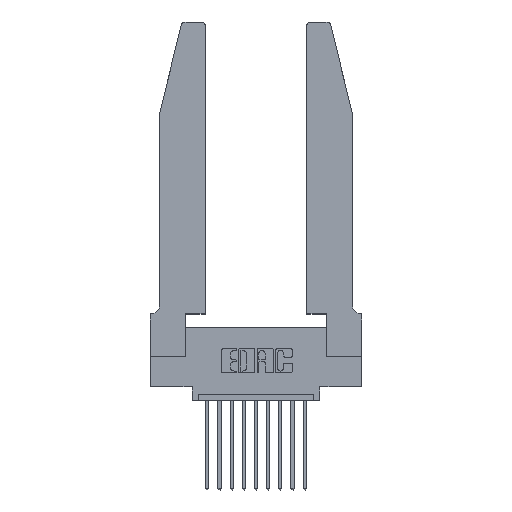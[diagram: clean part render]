
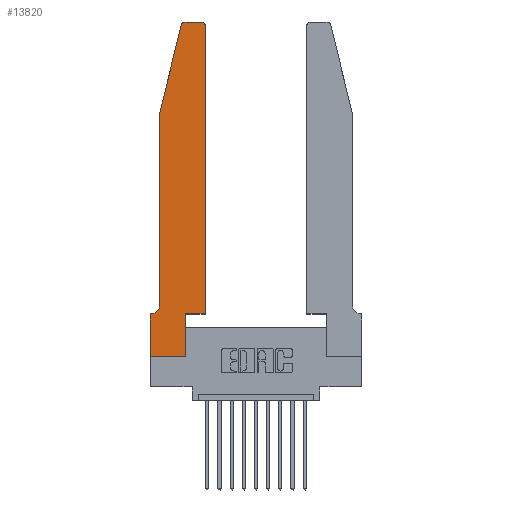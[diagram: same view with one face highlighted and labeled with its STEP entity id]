
A CAD part, top view. The second image highlights one B-rep face of the part: STEP entity #13820.
In plain terms, the highlighted planar face has unit normal (0, 0, 1).
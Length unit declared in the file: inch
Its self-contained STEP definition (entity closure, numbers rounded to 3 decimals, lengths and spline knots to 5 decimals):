
#143 = EDGE_CURVE ( 'NONE', #6618, #10646, #12908, .T. ) ;
#190 = ORIENTED_EDGE ( 'NONE', *, *, #7214, .T. ) ;
#289 = ORIENTED_EDGE ( 'NONE', *, *, #8067, .T. ) ;
#388 = CARTESIAN_POINT ( 'NONE',  ( 0.2865, 0.35, 0.37 ) ) ;
#455 = LINE ( 'NONE', #8012, #11568 ) ;
#609 = CARTESIAN_POINT ( 'NONE',  ( 0.0755, 2., 0.37 ) ) ;
#810 = LINE ( 'NONE', #609, #11160 ) ;
#1087 = VERTEX_POINT ( 'NONE', #6356 ) ;
#1095 = DIRECTION ( 'NONE',  ( -1., 0., 0. ) ) ;
#1259 = ORIENTED_EDGE ( 'NONE', *, *, #8394, .T. ) ;
#1332 = ORIENTED_EDGE ( 'NONE', *, *, #14107, .T. ) ;
#1530 = LINE ( 'NONE', #13356, #5033 ) ;
#1899 = EDGE_CURVE ( 'NONE', #15328, #15574, #11701, .T. ) ;
#1963 = VECTOR ( 'NONE', #5445, 39.37008 ) ;
#1976 = VECTOR ( 'NONE', #10586, 39.37008 ) ;
#2927 = CARTESIAN_POINT ( 'NONE',  ( 0.0055, 0.35, 0.37 ) ) ;
#2948 = ORIENTED_EDGE ( 'NONE', *, *, #13200, .T. ) ;
#3394 = EDGE_CURVE ( 'NONE', #10646, #1087, #8757, .T. ) ;
#3444 = ORIENTED_EDGE ( 'NONE', *, *, #10690, .T. ) ;
#3724 = CARTESIAN_POINT ( 'NONE',  ( 0.4205, 2.72, 0.37 ) ) ;
#3927 = VECTOR ( 'NONE', #7166, 39.37008 ) ;
#3982 = ORIENTED_EDGE ( 'NONE', *, *, #9500, .T. ) ;
#4256 = CARTESIAN_POINT ( 'NONE',  ( 0., 0., 0.37 ) ) ;
#4300 = CARTESIAN_POINT ( 'NONE',  ( 0.2605, 2.75, 0.37 ) ) ;
#4341 = ORIENTED_EDGE ( 'NONE', *, *, #1899, .T. ) ;
#4399 = VERTEX_POINT ( 'NONE', #6681 ) ;
#4404 = DIRECTION ( 'NONE',  ( -1., 0., 0. ) ) ;
#5033 = VECTOR ( 'NONE', #12233, 39.37008 ) ;
#5445 = DIRECTION ( 'NONE',  ( 0., 1., 0. ) ) ;
#5549 = VERTEX_POINT ( 'NONE', #4256 ) ;
#5720 = AXIS2_PLACEMENT_3D ( 'NONE', #7380, #11076, #8801 ) ;
#5830 = DIRECTION ( 'NONE',  ( 0., 0., 1. ) ) ;
#6044 = ORIENTED_EDGE ( 'NONE', *, *, #8778, .T. ) ;
#6047 = DIRECTION ( 'NONE',  ( 1., 0., 0. ) ) ;
#6051 = CARTESIAN_POINT ( 'NONE',  ( 0., 0.35, 0.37 ) ) ;
#6344 = CARTESIAN_POINT ( 'NONE',  ( 0.4505, 0.35, 0.37 ) ) ;
#6356 = CARTESIAN_POINT ( 'NONE',  ( 0.25487, 2.72718, 0.37 ) ) ;
#6618 = VERTEX_POINT ( 'NONE', #15232 ) ;
#6681 = CARTESIAN_POINT ( 'NONE',  ( 0.0755, 2., 0.37 ) ) ;
#6693 = DIRECTION ( 'NONE',  ( 1., 0., 0. ) ) ;
#6873 = VERTEX_POINT ( 'NONE', #14877 ) ;
#7014 = CARTESIAN_POINT ( 'NONE',  ( 0.0755, 0.42, 0.37 ) ) ;
#7020 = VERTEX_POINT ( 'NONE', #2927 ) ;
#7166 = DIRECTION ( 'NONE',  ( 1., 0., 0. ) ) ;
#7214 = EDGE_CURVE ( 'NONE', #4399, #14299, #810, .T. ) ;
#7265 = LINE ( 'NONE', #388, #7478 ) ;
#7380 = CARTESIAN_POINT ( 'NONE',  ( 0., 0.35, 0.37 ) ) ;
#7478 = VECTOR ( 'NONE', #10093, 39.37008 ) ;
#7617 = CIRCLE ( 'NONE', #12773, 0.03 ) ;
#7689 = EDGE_CURVE ( 'NONE', #7020, #16111, #13285, .T. ) ;
#7711 = VERTEX_POINT ( 'NONE', #15717 ) ;
#8012 = CARTESIAN_POINT ( 'NONE',  ( 0., 0., 0.37 ) ) ;
#8067 = EDGE_CURVE ( 'NONE', #7711, #15328, #9184, .T. ) ;
#8142 = CIRCLE ( 'NONE', #8944, 0.07 ) ;
#8385 = EDGE_LOOP ( 'NONE', ( #15115, #14340, #6044, #190, #3444, #8931, #3982, #1332, #2948, #289, #4341, #1259 ) ) ;
#8394 = EDGE_CURVE ( 'NONE', #15574, #6618, #7617, .T. ) ;
#8757 = CIRCLE ( 'NONE', #11583, 0.03 ) ;
#8778 = EDGE_CURVE ( 'NONE', #1087, #4399, #14838, .T. ) ;
#8801 = DIRECTION ( 'NONE',  ( 1., 0., 0. ) ) ;
#8931 = ORIENTED_EDGE ( 'NONE', *, *, #7689, .T. ) ;
#8944 = AXIS2_PLACEMENT_3D ( 'NONE', #14574, #9771, #1095 ) ;
#9184 = LINE ( 'NONE', #15955, #3927 ) ;
#9376 = CARTESIAN_POINT ( 'NONE',  ( 0.0755, 0.35, 0.37 ) ) ;
#9500 = EDGE_CURVE ( 'NONE', #16111, #5549, #1530, .T. ) ;
#9771 = DIRECTION ( 'NONE',  ( 0., 0., -1. ) ) ;
#9834 = DIRECTION ( 'NONE',  ( -0.239, -0.971, 0. ) ) ;
#10093 = DIRECTION ( 'NONE',  ( 0., 1., 0. ) ) ;
#10586 = DIRECTION ( 'NONE',  ( -1., 0., 0. ) ) ;
#10645 = CARTESIAN_POINT ( 'NONE',  ( 0.4505, 2.72, 0.37 ) ) ;
#10646 = VERTEX_POINT ( 'NONE', #10950 ) ;
#10690 = EDGE_CURVE ( 'NONE', #14299, #7020, #8142, .T. ) ;
#10950 = CARTESIAN_POINT ( 'NONE',  ( 0.284, 2.75, 0.37 ) ) ;
#11076 = DIRECTION ( 'NONE',  ( 0., 0., 1. ) ) ;
#11160 = VECTOR ( 'NONE', #11981, 39.37008 ) ;
#11568 = VECTOR ( 'NONE', #6693, 39.37008 ) ;
#11583 = AXIS2_PLACEMENT_3D ( 'NONE', #14567, #5830, #16027 ) ;
#11701 = LINE ( 'NONE', #12835, #1963 ) ;
#11981 = DIRECTION ( 'NONE',  ( 0., -1., 0. ) ) ;
#12233 = DIRECTION ( 'NONE',  ( 0., -1., 0. ) ) ;
#12773 = AXIS2_PLACEMENT_3D ( 'NONE', #3724, #14784, #6047 ) ;
#12835 = CARTESIAN_POINT ( 'NONE',  ( 0.4505, 0.35, 0.37 ) ) ;
#12908 = LINE ( 'NONE', #4300, #1976 ) ;
#13200 = EDGE_CURVE ( 'NONE', #6873, #7711, #7265, .T. ) ;
#13285 = LINE ( 'NONE', #9376, #14865 ) ;
#13356 = CARTESIAN_POINT ( 'NONE',  ( 0., 0., 0.37 ) ) ;
#13820 = ADVANCED_FACE ( 'NONE', ( #16044 ), #15016, .T. ) ;
#14059 = VECTOR ( 'NONE', #9834, 39.37008 ) ;
#14107 = EDGE_CURVE ( 'NONE', #5549, #6873, #455, .T. ) ;
#14299 = VERTEX_POINT ( 'NONE', #7014 ) ;
#14340 = ORIENTED_EDGE ( 'NONE', *, *, #3394, .T. ) ;
#14567 = CARTESIAN_POINT ( 'NONE',  ( 0.284, 2.72, 0.37 ) ) ;
#14574 = CARTESIAN_POINT ( 'NONE',  ( 0.0055, 0.42, 0.37 ) ) ;
#14784 = DIRECTION ( 'NONE',  ( 0., 0., 1. ) ) ;
#14838 = LINE ( 'NONE', #16034, #14059 ) ;
#14865 = VECTOR ( 'NONE', #4404, 39.37008 ) ;
#14877 = CARTESIAN_POINT ( 'NONE',  ( 0.2865, 0., 0.37 ) ) ;
#15016 = PLANE ( 'NONE',  #5720 ) ;
#15115 = ORIENTED_EDGE ( 'NONE', *, *, #143, .T. ) ;
#15232 = CARTESIAN_POINT ( 'NONE',  ( 0.4205, 2.75, 0.37 ) ) ;
#15328 = VERTEX_POINT ( 'NONE', #6344 ) ;
#15574 = VERTEX_POINT ( 'NONE', #10645 ) ;
#15717 = CARTESIAN_POINT ( 'NONE',  ( 0.2865, 0.35, 0.37 ) ) ;
#15955 = CARTESIAN_POINT ( 'NONE',  ( 0.4505, 0.35, 0.37 ) ) ;
#16027 = DIRECTION ( 'NONE',  ( 1., 0., 0. ) ) ;
#16034 = CARTESIAN_POINT ( 'NONE',  ( 0.0755, 2., 0.37 ) ) ;
#16044 = FACE_OUTER_BOUND ( 'NONE', #8385, .T. ) ;
#16111 = VERTEX_POINT ( 'NONE', #6051 ) ;
